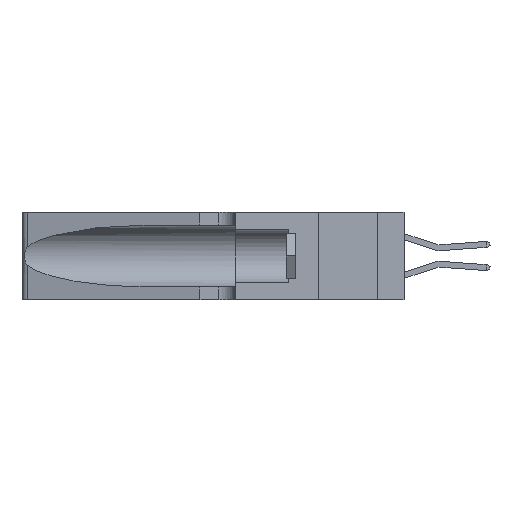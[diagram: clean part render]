
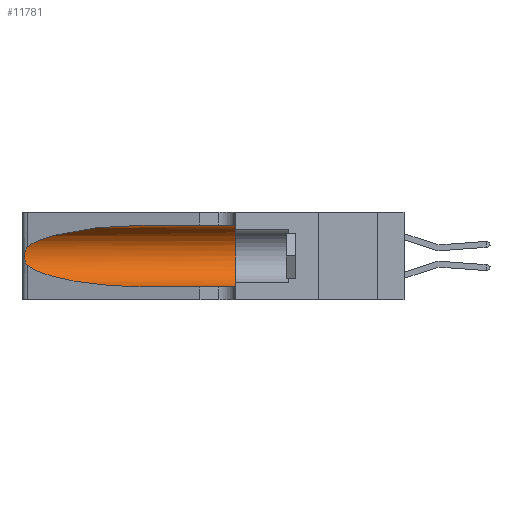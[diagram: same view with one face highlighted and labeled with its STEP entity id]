
A CAD part, left-side view. The second image highlights one B-rep face of the part: STEP entity #11781.
In plain terms, the highlighted cylindrical face has radius 3.308 mm (diameter 6.617 mm), a partial arc.
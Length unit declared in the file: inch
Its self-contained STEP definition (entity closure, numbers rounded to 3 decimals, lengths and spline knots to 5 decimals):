
#267 = LINE ( 'NONE', #8443, #6261 ) ;
#741 = CARTESIAN_POINT ( 'NONE',  ( 0.1305, 0.35, 0.05475 ) ) ;
#2238 = EDGE_CURVE ( 'NONE', #2888, #42867, #21743, .T. ) ;
#2369 = AXIS2_PLACEMENT_3D ( 'NONE', #2858, #24022, #24305 ) ;
#2858 = CARTESIAN_POINT ( 'NONE',  ( 0.1305, 0.35, 0.185 ) ) ;
#2888 = VERTEX_POINT ( 'NONE', #40676 ) ;
#2972 = CARTESIAN_POINT ( 'NONE',  ( 0.25854, 1.2359, 0.20912 ) ) ;
#6140 = VERTEX_POINT ( 'NONE', #42012 ) ;
#6261 = VECTOR ( 'NONE', #32414, 39.37008 ) ;
#6322 = CARTESIAN_POINT ( 'NONE',  ( 0.25789, 1.23486, 0.15765 ) ) ;
#6470 = CARTESIAN_POINT ( 'NONE',  ( 0.25856, 1.23593, 0.16098 ) ) ;
#6850 = CARTESIAN_POINT ( 'NONE',  ( 0.2373, 1.15595, 0.28018 ) ) ;
#7086 = FACE_OUTER_BOUND ( 'NONE', #25610, .T. ) ;
#8443 = CARTESIAN_POINT ( 'NONE',  ( 0.1305, 1.61858, 0.31525 ) ) ;
#9013 = EDGE_CURVE ( 'NONE', #6140, #18915, #267, .T. ) ;
#10001 = DIRECTION ( 'NONE',  ( 0., 0., -1. ) ) ;
#10374 = EDGE_CURVE ( 'NONE', #6140, #18745, #17334, .T. ) ;
#10742 =( BOUNDED_CURVE ( )  B_SPLINE_CURVE ( 3, ( #26610, #41632, #20848, #17718 ),
 .UNSPECIFIED., .F., .F. ) 
 B_SPLINE_CURVE_WITH_KNOTS ( ( 4, 4 ),
 ( 3.44316, 4.71239 ),
 .UNSPECIFIED. ) 
 CURVE ( )  GEOMETRIC_REPRESENTATION_ITEM ( )  RATIONAL_B_SPLINE_CURVE ( ( 1., 0.87, 0.87, 1. ) ) 
 REPRESENTATION_ITEM ( '' )  );
#11035 = ORIENTED_EDGE ( 'NONE', *, *, #42474, .T. ) ;
#11300 = CARTESIAN_POINT ( 'NONE',  ( 0.1305, 1.61858, 0.05475 ) ) ;
#11781 = ADVANCED_FACE ( 'NONE', ( #7086 ), #32855, .F. ) ;
#12110 = ORIENTED_EDGE ( 'NONE', *, *, #27845, .F. ) ;
#13086 = CARTESIAN_POINT ( 'NONE',  ( 0.25487, 1.22718, 0.22369 ) ) ;
#13517 = CARTESIAN_POINT ( 'NONE',  ( 0.26017, 1.23833, 0.17102 ) ) ;
#14333 = AXIS2_PLACEMENT_3D ( 'NONE', #23062, #20178, #10001 ) ;
#16658 = CARTESIAN_POINT ( 'NONE',  ( 0.25639, 1.23186, 0.15144 ) ) ;
#17334 =( BOUNDED_CURVE ( )  B_SPLINE_CURVE ( 3, ( #27410, #41051, #6850, #20330 ),
 .UNSPECIFIED., .F., .F. ) 
 B_SPLINE_CURVE_WITH_KNOTS ( ( 4, 4 ),
 ( 1.5708, 2.84003 ),
 .UNSPECIFIED. ) 
 CURVE ( )  GEOMETRIC_REPRESENTATION_ITEM ( )  RATIONAL_B_SPLINE_CURVE ( ( 1., 0.87, 0.87, 1. ) ) 
 REPRESENTATION_ITEM ( '' )  );
#17573 = B_SPLINE_CURVE_WITH_KNOTS ( 'NONE', 3,
 ( #13086, #44111, #33764, #43953, #2972, #24002, #20534, #37233, #13517, #6470, #6322, #16658, #44249, #30444 ),
 .UNSPECIFIED., .F., .F.,
 ( 4, 2, 2, 2, 2, 2, 4 ),
 ( 0., 0.00027, 0.00053, 0.00107, 0.0016, 0.00187, 0.00214 ),
 .UNSPECIFIED. ) ;
#17718 = CARTESIAN_POINT ( 'NONE',  ( 0.1305, 0.72297, 0.05475 ) ) ;
#17956 = VECTOR ( 'NONE', #24941, 39.37008 ) ;
#18745 = VERTEX_POINT ( 'NONE', #29730 ) ;
#18915 = VERTEX_POINT ( 'NONE', #22996 ) ;
#19650 = ORIENTED_EDGE ( 'NONE', *, *, #9013, .F. ) ;
#20178 = DIRECTION ( 'NONE',  ( 0., -1., 0. ) ) ;
#20330 = CARTESIAN_POINT ( 'NONE',  ( 0.25487, 1.22718, 0.22369 ) ) ;
#20534 = CARTESIAN_POINT ( 'NONE',  ( 0.26075, 1.23896, 0.19203 ) ) ;
#20848 = CARTESIAN_POINT ( 'NONE',  ( 0.18966, 0.96281, 0.05475 ) ) ;
#21743 = LINE ( 'NONE', #11300, #17956 ) ;
#22996 = CARTESIAN_POINT ( 'NONE',  ( 0.1305, 0.35, 0.31525 ) ) ;
#23062 = CARTESIAN_POINT ( 'NONE',  ( 0.1305, 1.61858, 0.185 ) ) ;
#24002 = CARTESIAN_POINT ( 'NONE',  ( 0.26018, 1.23835, 0.19895 ) ) ;
#24022 = DIRECTION ( 'NONE',  ( 0., 1., 0. ) ) ;
#24305 = DIRECTION ( 'NONE',  ( 0., 0., 1. ) ) ;
#24941 = DIRECTION ( 'NONE',  ( 0., -1., 0. ) ) ;
#25610 = EDGE_LOOP ( 'NONE', ( #27542, #11035, #35152, #38919, #12110, #19650 ) ) ;
#26610 = CARTESIAN_POINT ( 'NONE',  ( 0.25487, 1.22718, 0.14631 ) ) ;
#27277 = EDGE_CURVE ( 'NONE', #29877, #2888, #10742, .T. ) ;
#27410 = CARTESIAN_POINT ( 'NONE',  ( 0.1305, 0.72297, 0.31525 ) ) ;
#27542 = ORIENTED_EDGE ( 'NONE', *, *, #10374, .T. ) ;
#27845 = EDGE_CURVE ( 'NONE', #18915, #42867, #39415, .T. ) ;
#29730 = CARTESIAN_POINT ( 'NONE',  ( 0.25487, 1.22718, 0.22369 ) ) ;
#29877 = VERTEX_POINT ( 'NONE', #41957 ) ;
#30444 = CARTESIAN_POINT ( 'NONE',  ( 0.25487, 1.22718, 0.14631 ) ) ;
#32414 = DIRECTION ( 'NONE',  ( 0., -1., 0. ) ) ;
#32855 = CYLINDRICAL_SURFACE ( 'NONE', #14333, 0.13025 ) ;
#33764 = CARTESIAN_POINT ( 'NONE',  ( 0.25639, 1.23184, 0.21858 ) ) ;
#35152 = ORIENTED_EDGE ( 'NONE', *, *, #27277, .T. ) ;
#37233 = CARTESIAN_POINT ( 'NONE',  ( 0.26075, 1.23896, 0.178 ) ) ;
#38919 = ORIENTED_EDGE ( 'NONE', *, *, #2238, .T. ) ;
#39415 = CIRCLE ( 'NONE', #2369, 0.13025 ) ;
#40676 = CARTESIAN_POINT ( 'NONE',  ( 0.1305, 0.72297, 0.05475 ) ) ;
#41051 = CARTESIAN_POINT ( 'NONE',  ( 0.18966, 0.96281, 0.31525 ) ) ;
#41632 = CARTESIAN_POINT ( 'NONE',  ( 0.2373, 1.15595, 0.08982 ) ) ;
#41957 = CARTESIAN_POINT ( 'NONE',  ( 0.25487, 1.22718, 0.14631 ) ) ;
#42012 = CARTESIAN_POINT ( 'NONE',  ( 0.1305, 0.72297, 0.31525 ) ) ;
#42474 = EDGE_CURVE ( 'NONE', #18745, #29877, #17573, .T. ) ;
#42867 = VERTEX_POINT ( 'NONE', #741 ) ;
#43953 = CARTESIAN_POINT ( 'NONE',  ( 0.25787, 1.23484, 0.2124 ) ) ;
#44111 = CARTESIAN_POINT ( 'NONE',  ( 0.25555, 1.22994, 0.2215 ) ) ;
#44249 = CARTESIAN_POINT ( 'NONE',  ( 0.25555, 1.22993, 0.14849 ) ) ;
